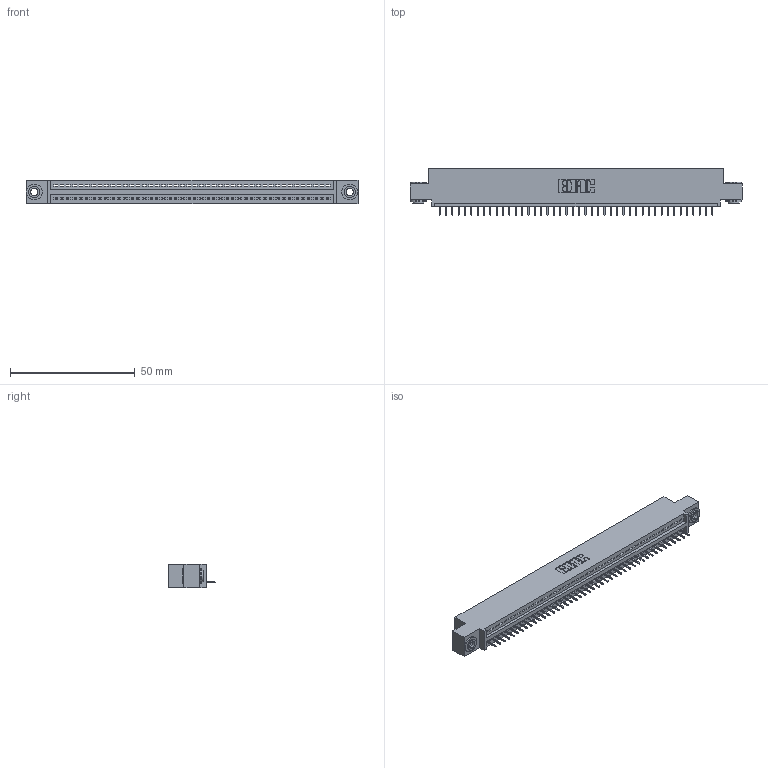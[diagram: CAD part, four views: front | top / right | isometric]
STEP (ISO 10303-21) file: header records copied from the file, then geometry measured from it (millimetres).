
FILE_DESCRIPTION (( 'STEP AP203' ), '1' );
FILE_NAME ('845-044-525-403.STEP', '2020-09-23T06:38:51', ( '' ), ( '' ), 'SwSTEP 2.0', 'SolidWorks 2020', '' );
FILE_SCHEMA (( 'CONFIG_CONTROL_DESIGN' ));
Length unit declared in the file: inch
Products named in the file (4): 345-292-001_345-293-125; 845-044-525-403; 845 Part_0.110 Offset - 0.156 Dia-TH; 345-250-002_345-250-002-102
Assembly tree (47 placements, depth 2):
  845-044-525-403
    845 Part_0.110 Offset - 0.156 Dia-TH
    345-292-001_345-293-125  x44
    345-250-002_345-250-002-102  x2
Bounding box: 132.97 x 18.72 x 9.4 mm (x, y, z)
Volume: 12412.3 mm3; surface area: 16219.3 mm2
Topology: 47 solids, 47 shells, 2896 faces, 8349 edges, 5386 vertices
Faces by surface type: plane 2118, cylinder 770, cone 8
Entity records: 33702 total; most frequent: CARTESIAN_POINT 5815, ORIENTED_EDGE 5786, DIRECTION 5107, EDGE_CURVE 2893, VECTOR 2565, LINE 2565, VERTEX_POINT 1922, AXIS2_PLACEMENT_3D 1271
